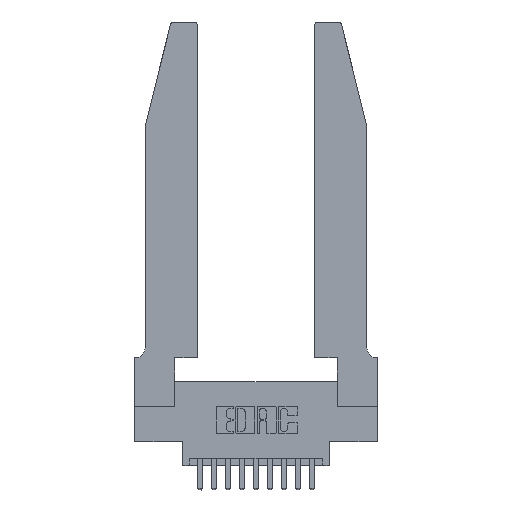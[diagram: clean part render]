
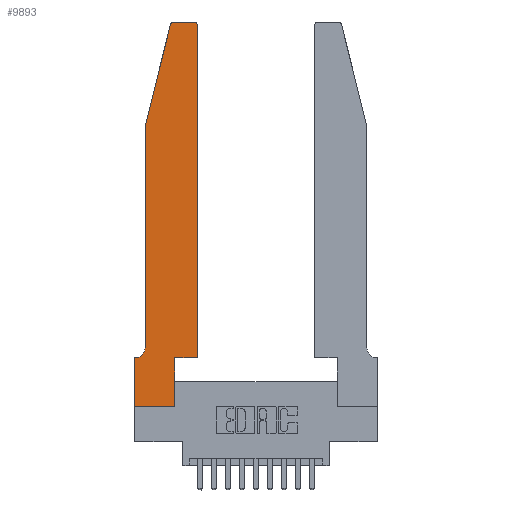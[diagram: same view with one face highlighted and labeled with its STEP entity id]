
A CAD part, top view. The second image highlights one B-rep face of the part: STEP entity #9893.
In plain terms, the highlighted planar face has unit normal (0, 0, 1).
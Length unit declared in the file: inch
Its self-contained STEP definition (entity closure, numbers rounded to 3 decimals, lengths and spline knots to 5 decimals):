
#418 = ORIENTED_EDGE ( 'NONE', *, *, #11103, .T. ) ;
#514 = CARTESIAN_POINT ( 'NONE',  ( 0.0755, 0.35, 0.37 ) ) ;
#1039 = VERTEX_POINT ( 'NONE', #15808 ) ;
#1133 = VERTEX_POINT ( 'NONE', #16062 ) ;
#1304 = CARTESIAN_POINT ( 'NONE',  ( 0., 0., 0.37 ) ) ;
#1334 = VECTOR ( 'NONE', #1919, 39.37008 ) ;
#1617 = CARTESIAN_POINT ( 'NONE',  ( 0.2865, 0.35, 0.37 ) ) ;
#1660 = ORIENTED_EDGE ( 'NONE', *, *, #14263, .T. ) ;
#1714 = VERTEX_POINT ( 'NONE', #14761 ) ;
#1919 = DIRECTION ( 'NONE',  ( -1., 0., 0. ) ) ;
#2124 = LINE ( 'NONE', #8784, #7898 ) ;
#2147 = CIRCLE ( 'NONE', #7665, 0.03 ) ;
#2166 = VECTOR ( 'NONE', #9375, 39.37008 ) ;
#2727 = LINE ( 'NONE', #514, #1334 ) ;
#2874 = CARTESIAN_POINT ( 'NONE',  ( 0.4205, 2.75, 0.37 ) ) ;
#3676 = DIRECTION ( 'NONE',  ( 0., 1., 0. ) ) ;
#3679 = CARTESIAN_POINT ( 'NONE',  ( 0.2605, 2.75, 0.37 ) ) ;
#3711 = CARTESIAN_POINT ( 'NONE',  ( 0., 0.35, 0.37 ) ) ;
#3718 = VERTEX_POINT ( 'NONE', #12216 ) ;
#3781 = CARTESIAN_POINT ( 'NONE',  ( 0.284, 2.75, 0.37 ) ) ;
#3885 = CIRCLE ( 'NONE', #9984, 0.07 ) ;
#3932 = LINE ( 'NONE', #13788, #7301 ) ;
#3937 = VECTOR ( 'NONE', #10803, 39.37008 ) ;
#4215 = CARTESIAN_POINT ( 'NONE',  ( 0.0755, 0.42, 0.37 ) ) ;
#4875 = VERTEX_POINT ( 'NONE', #3781 ) ;
#4933 = EDGE_CURVE ( 'NONE', #3718, #1039, #12341, .T. ) ;
#4972 = DIRECTION ( 'NONE',  ( 1., 0., 0. ) ) ;
#4988 = VECTOR ( 'NONE', #11365, 39.37008 ) ;
#4991 = DIRECTION ( 'NONE',  ( 0., 0., 1. ) ) ;
#5040 = ORIENTED_EDGE ( 'NONE', *, *, #5936, .T. ) ;
#5088 = ORIENTED_EDGE ( 'NONE', *, *, #13467, .T. ) ;
#5089 = DIRECTION ( 'NONE',  ( 1., 0., 0. ) ) ;
#5327 = CIRCLE ( 'NONE', #10211, 0.03 ) ;
#5468 = ORIENTED_EDGE ( 'NONE', *, *, #15348, .T. ) ;
#5779 = CARTESIAN_POINT ( 'NONE',  ( 0.0755, 2., 0.37 ) ) ;
#5796 = LINE ( 'NONE', #3679, #4988 ) ;
#5936 = EDGE_CURVE ( 'NONE', #12955, #1133, #2727, .T. ) ;
#6373 = DIRECTION ( 'NONE',  ( 0., -1., 0. ) ) ;
#6401 = VECTOR ( 'NONE', #6373, 39.37008 ) ;
#7301 = VECTOR ( 'NONE', #3676, 39.37008 ) ;
#7591 = PLANE ( 'NONE',  #15776 ) ;
#7630 = EDGE_LOOP ( 'NONE', ( #418, #5468, #14753, #13385, #15860, #5040, #12807, #8590, #8120, #1660, #5088, #15568 ) ) ;
#7665 = AXIS2_PLACEMENT_3D ( 'NONE', #12874, #14126, #15362 ) ;
#7898 = VECTOR ( 'NONE', #10056, 39.37008 ) ;
#8120 = ORIENTED_EDGE ( 'NONE', *, *, #11939, .T. ) ;
#8460 = VERTEX_POINT ( 'NONE', #11493 ) ;
#8518 = EDGE_CURVE ( 'NONE', #11448, #12955, #3885, .T. ) ;
#8590 = ORIENTED_EDGE ( 'NONE', *, *, #4933, .T. ) ;
#8784 = CARTESIAN_POINT ( 'NONE',  ( 0.0755, 2., 0.37 ) ) ;
#8915 = LINE ( 'NONE', #5779, #3937 ) ;
#9375 = DIRECTION ( 'NONE',  ( 1., 0., 0. ) ) ;
#9395 = FACE_OUTER_BOUND ( 'NONE', #7630, .T. ) ;
#9486 = DIRECTION ( 'NONE',  ( 0., 0., -1. ) ) ;
#9893 = ADVANCED_FACE ( 'NONE', ( #9395 ), #7591, .T. ) ;
#9984 = AXIS2_PLACEMENT_3D ( 'NONE', #14474, #9486, #13221 ) ;
#10056 = DIRECTION ( 'NONE',  ( 0., -1., 0. ) ) ;
#10166 = VERTEX_POINT ( 'NONE', #11872 ) ;
#10211 = AXIS2_PLACEMENT_3D ( 'NONE', #14950, #4991, #12594 ) ;
#10598 = CARTESIAN_POINT ( 'NONE',  ( 0., 0., 0.37 ) ) ;
#10732 = VECTOR ( 'NONE', #5089, 39.37008 ) ;
#10803 = DIRECTION ( 'NONE',  ( -0.239, -0.971, 0. ) ) ;
#10893 = EDGE_CURVE ( 'NONE', #1133, #3718, #11981, .T. ) ;
#10975 = CARTESIAN_POINT ( 'NONE',  ( 0.25487, 2.72718, 0.37 ) ) ;
#11103 = EDGE_CURVE ( 'NONE', #15655, #4875, #5796, .T. ) ;
#11365 = DIRECTION ( 'NONE',  ( -1., 0., 0. ) ) ;
#11405 = CARTESIAN_POINT ( 'NONE',  ( 0.0055, 0.35, 0.37 ) ) ;
#11448 = VERTEX_POINT ( 'NONE', #4215 ) ;
#11493 = CARTESIAN_POINT ( 'NONE',  ( 0.0755, 2., 0.37 ) ) ;
#11545 = VECTOR ( 'NONE', #15755, 39.37008 ) ;
#11716 = LINE ( 'NONE', #12734, #10732 ) ;
#11872 = CARTESIAN_POINT ( 'NONE',  ( 0.2865, 0.35, 0.37 ) ) ;
#11939 = EDGE_CURVE ( 'NONE', #1039, #10166, #13140, .T. ) ;
#11981 = LINE ( 'NONE', #1304, #6401 ) ;
#12216 = CARTESIAN_POINT ( 'NONE',  ( 0., 0., 0.37 ) ) ;
#12341 = LINE ( 'NONE', #10598, #2166 ) ;
#12594 = DIRECTION ( 'NONE',  ( 1., 0., 0. ) ) ;
#12625 = DIRECTION ( 'NONE',  ( 0., 0., 1. ) ) ;
#12734 = CARTESIAN_POINT ( 'NONE',  ( 0.4505, 0.35, 0.37 ) ) ;
#12807 = ORIENTED_EDGE ( 'NONE', *, *, #10893, .T. ) ;
#12874 = CARTESIAN_POINT ( 'NONE',  ( 0.4205, 2.72, 0.37 ) ) ;
#12955 = VERTEX_POINT ( 'NONE', #11405 ) ;
#13140 = LINE ( 'NONE', #1617, #11545 ) ;
#13221 = DIRECTION ( 'NONE',  ( -1., 0., 0. ) ) ;
#13261 = EDGE_CURVE ( 'NONE', #14712, #8460, #8915, .T. ) ;
#13339 = VERTEX_POINT ( 'NONE', #13613 ) ;
#13385 = ORIENTED_EDGE ( 'NONE', *, *, #15403, .T. ) ;
#13467 = EDGE_CURVE ( 'NONE', #13339, #1714, #3932, .T. ) ;
#13613 = CARTESIAN_POINT ( 'NONE',  ( 0.4505, 0.35, 0.37 ) ) ;
#13788 = CARTESIAN_POINT ( 'NONE',  ( 0.4505, 0.35, 0.37 ) ) ;
#14126 = DIRECTION ( 'NONE',  ( 0., 0., 1. ) ) ;
#14263 = EDGE_CURVE ( 'NONE', #10166, #13339, #11716, .T. ) ;
#14474 = CARTESIAN_POINT ( 'NONE',  ( 0.0055, 0.42, 0.37 ) ) ;
#14712 = VERTEX_POINT ( 'NONE', #10975 ) ;
#14753 = ORIENTED_EDGE ( 'NONE', *, *, #13261, .T. ) ;
#14761 = CARTESIAN_POINT ( 'NONE',  ( 0.4505, 2.72, 0.37 ) ) ;
#14950 = CARTESIAN_POINT ( 'NONE',  ( 0.284, 2.72, 0.37 ) ) ;
#14966 = EDGE_CURVE ( 'NONE', #1714, #15655, #2147, .T. ) ;
#15348 = EDGE_CURVE ( 'NONE', #4875, #14712, #5327, .T. ) ;
#15362 = DIRECTION ( 'NONE',  ( 1., 0., 0. ) ) ;
#15403 = EDGE_CURVE ( 'NONE', #8460, #11448, #2124, .T. ) ;
#15568 = ORIENTED_EDGE ( 'NONE', *, *, #14966, .T. ) ;
#15655 = VERTEX_POINT ( 'NONE', #2874 ) ;
#15755 = DIRECTION ( 'NONE',  ( 0., 1., 0. ) ) ;
#15776 = AXIS2_PLACEMENT_3D ( 'NONE', #3711, #12625, #4972 ) ;
#15808 = CARTESIAN_POINT ( 'NONE',  ( 0.2865, 0., 0.37 ) ) ;
#15860 = ORIENTED_EDGE ( 'NONE', *, *, #8518, .T. ) ;
#16062 = CARTESIAN_POINT ( 'NONE',  ( 0., 0.35, 0.37 ) ) ;
